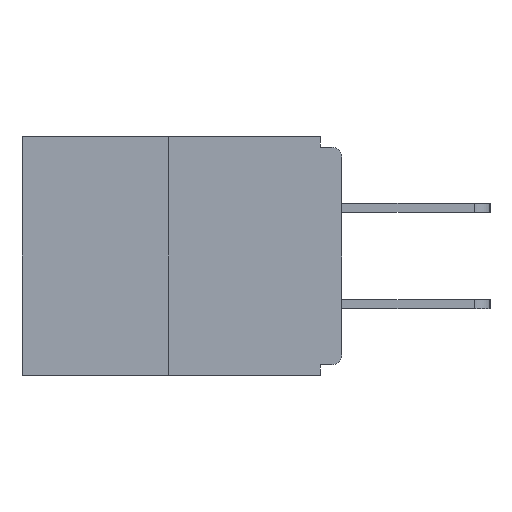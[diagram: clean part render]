
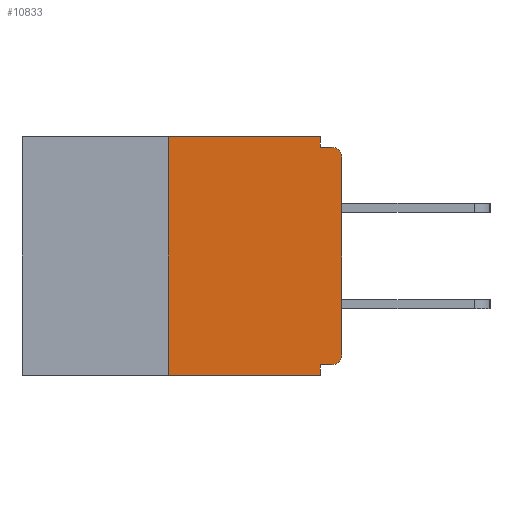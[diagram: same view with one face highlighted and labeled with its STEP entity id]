
A CAD part, left-side view. The second image highlights one B-rep face of the part: STEP entity #10833.
In plain terms, the highlighted planar face has unit normal (-1, 0, 0).
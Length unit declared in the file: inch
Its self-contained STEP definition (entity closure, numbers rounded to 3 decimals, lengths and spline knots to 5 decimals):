
#17 = ORIENTED_EDGE ( 'NONE', *, *, #4774, .T. ) ;
#292 = EDGE_CURVE ( 'NONE', #5981, #7159, #8497, .T. ) ;
#426 = CARTESIAN_POINT ( 'NONE',  ( 0., 0., -0.328 ) ) ;
#669 = VERTEX_POINT ( 'NONE', #8256 ) ;
#780 = CARTESIAN_POINT ( 'NONE',  ( 0., 0., 0. ) ) ;
#797 = DIRECTION ( 'NONE',  ( 0., 0., -1. ) ) ;
#1089 = CARTESIAN_POINT ( 'NONE',  ( 0., 0.031, -0.328 ) ) ;
#1329 = CARTESIAN_POINT ( 'NONE',  ( 0., 0.46, 0. ) ) ;
#1749 = ORIENTED_EDGE ( 'NONE', *, *, #5441, .F. ) ;
#2180 = ORIENTED_EDGE ( 'NONE', *, *, #4377, .F. ) ;
#2278 = CARTESIAN_POINT ( 'NONE',  ( 0., 0.031, -0.343 ) ) ;
#2692 = VERTEX_POINT ( 'NONE', #3064 ) ;
#2715 = AXIS2_PLACEMENT_3D ( 'NONE', #4232, #9411, #11627 ) ;
#3044 = CARTESIAN_POINT ( 'NONE',  ( 0., 0.015, -0.03 ) ) ;
#3064 = CARTESIAN_POINT ( 'NONE',  ( 0., 0.25, -0.343 ) ) ;
#3143 = DIRECTION ( 'NONE',  ( 0., -1., 0. ) ) ;
#3609 = VECTOR ( 'NONE', #5861, 39.37008 ) ;
#3859 = CARTESIAN_POINT ( 'NONE',  ( 0., 0.25, 0. ) ) ;
#4183 = VERTEX_POINT ( 'NONE', #7226 ) ;
#4232 = CARTESIAN_POINT ( 'NONE',  ( 0., 0.015, -0.313 ) ) ;
#4347 = CARTESIAN_POINT ( 'NONE',  ( 0., 0.46, 0. ) ) ;
#4377 = EDGE_CURVE ( 'NONE', #2692, #6085, #9682, .T. ) ;
#4435 = EDGE_LOOP ( 'NONE', ( #10690, #2180, #7878, #1749, #9866, #6813, #6011, #17, #13465, #7876 ) ) ;
#4774 = EDGE_CURVE ( 'NONE', #7159, #7792, #12801, .T. ) ;
#5296 = CARTESIAN_POINT ( 'NONE',  ( 0., 0., -0.03 ) ) ;
#5441 = EDGE_CURVE ( 'NONE', #7714, #6295, #6858, .T. ) ;
#5861 = DIRECTION ( 'NONE',  ( 0., -1., 0. ) ) ;
#5948 = LINE ( 'NONE', #426, #9610 ) ;
#5981 = VERTEX_POINT ( 'NONE', #10332 ) ;
#6011 = ORIENTED_EDGE ( 'NONE', *, *, #292, .T. ) ;
#6085 = VERTEX_POINT ( 'NONE', #3859 ) ;
#6115 = AXIS2_PLACEMENT_3D ( 'NONE', #1329, #7701, #9401 ) ;
#6144 = DIRECTION ( 'NONE',  ( -1., 0., 0. ) ) ;
#6186 = DIRECTION ( 'NONE',  ( 0., 0., 1. ) ) ;
#6295 = VERTEX_POINT ( 'NONE', #2278 ) ;
#6420 = VECTOR ( 'NONE', #11956, 39.37008 ) ;
#6475 = DIRECTION ( 'NONE',  ( 0., -1., 0. ) ) ;
#6743 = CARTESIAN_POINT ( 'NONE',  ( 0., 0.031, 0. ) ) ;
#6813 = ORIENTED_EDGE ( 'NONE', *, *, #8291, .T. ) ;
#6858 = LINE ( 'NONE', #11388, #13585 ) ;
#7159 = VERTEX_POINT ( 'NONE', #5296 ) ;
#7226 = CARTESIAN_POINT ( 'NONE',  ( 0., 0.015, -0.328 ) ) ;
#7248 = LINE ( 'NONE', #13031, #3609 ) ;
#7494 = EDGE_CURVE ( 'NONE', #4183, #7714, #5948, .T. ) ;
#7654 = PLANE ( 'NONE',  #6115 ) ;
#7701 = DIRECTION ( 'NONE',  ( 1., 0., 0. ) ) ;
#7714 = VERTEX_POINT ( 'NONE', #1089 ) ;
#7792 = VERTEX_POINT ( 'NONE', #10952 ) ;
#7832 = CARTESIAN_POINT ( 'NONE',  ( 0., 0.031, -0.015 ) ) ;
#7866 = VERTEX_POINT ( 'NONE', #7832 ) ;
#7876 = ORIENTED_EDGE ( 'NONE', *, *, #11402, .F. ) ;
#7878 = ORIENTED_EDGE ( 'NONE', *, *, #9191, .T. ) ;
#7925 = LINE ( 'NONE', #6743, #6420 ) ;
#8256 = CARTESIAN_POINT ( 'NONE',  ( 0., 0.031, 0. ) ) ;
#8291 = EDGE_CURVE ( 'NONE', #4183, #5981, #8581, .T. ) ;
#8497 = LINE ( 'NONE', #780, #12148 ) ;
#8581 = CIRCLE ( 'NONE', #2715, 0.015 ) ;
#8599 = CARTESIAN_POINT ( 'NONE',  ( 0., 0., -0.015 ) ) ;
#9034 = LINE ( 'NONE', #4347, #12337 ) ;
#9190 = LINE ( 'NONE', #8599, #10379 ) ;
#9191 = EDGE_CURVE ( 'NONE', #2692, #6295, #7248, .T. ) ;
#9401 = DIRECTION ( 'NONE',  ( 0., 0., -1. ) ) ;
#9411 = DIRECTION ( 'NONE',  ( -1., 0., 0. ) ) ;
#9610 = VECTOR ( 'NONE', #9739, 39.37008 ) ;
#9682 = LINE ( 'NONE', #13384, #12437 ) ;
#9739 = DIRECTION ( 'NONE',  ( 0., 1., 0. ) ) ;
#9866 = ORIENTED_EDGE ( 'NONE', *, *, #7494, .F. ) ;
#10332 = CARTESIAN_POINT ( 'NONE',  ( 0., 0., -0.313 ) ) ;
#10379 = VECTOR ( 'NONE', #3143, 39.37008 ) ;
#10451 = DIRECTION ( 'NONE',  ( 0., 0., 1. ) ) ;
#10452 = EDGE_CURVE ( 'NONE', #7866, #7792, #9190, .T. ) ;
#10690 = ORIENTED_EDGE ( 'NONE', *, *, #12506, .F. ) ;
#10779 = AXIS2_PLACEMENT_3D ( 'NONE', #3044, #6144, #797 ) ;
#10833 = ADVANCED_FACE ( 'NONE', ( #12572 ), #7654, .F. ) ;
#10952 = CARTESIAN_POINT ( 'NONE',  ( 0., 0.015, -0.015 ) ) ;
#11388 = CARTESIAN_POINT ( 'NONE',  ( 0., 0.031, -0.343 ) ) ;
#11402 = EDGE_CURVE ( 'NONE', #669, #7866, #7925, .T. ) ;
#11627 = DIRECTION ( 'NONE',  ( 0., 0., -1. ) ) ;
#11956 = DIRECTION ( 'NONE',  ( 0., 0., -1. ) ) ;
#12148 = VECTOR ( 'NONE', #10451, 39.37008 ) ;
#12337 = VECTOR ( 'NONE', #6475, 39.37008 ) ;
#12437 = VECTOR ( 'NONE', #6186, 39.37008 ) ;
#12506 = EDGE_CURVE ( 'NONE', #6085, #669, #9034, .T. ) ;
#12572 = FACE_OUTER_BOUND ( 'NONE', #4435, .T. ) ;
#12801 = CIRCLE ( 'NONE', #10779, 0.015 ) ;
#13031 = CARTESIAN_POINT ( 'NONE',  ( 0., 0.46, -0.343 ) ) ;
#13384 = CARTESIAN_POINT ( 'NONE',  ( 0., 0.25, 0. ) ) ;
#13445 = DIRECTION ( 'NONE',  ( 0., 0., -1. ) ) ;
#13465 = ORIENTED_EDGE ( 'NONE', *, *, #10452, .F. ) ;
#13585 = VECTOR ( 'NONE', #13445, 39.37008 ) ;
